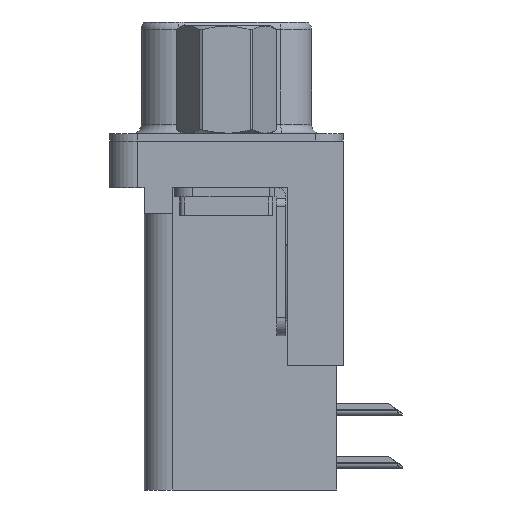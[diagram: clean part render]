
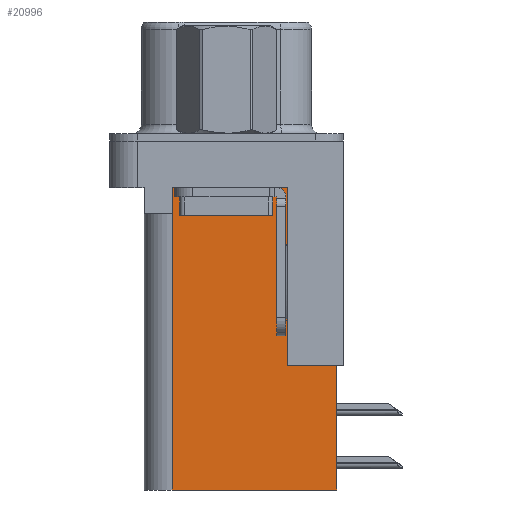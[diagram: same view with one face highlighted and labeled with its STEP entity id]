
A CAD part, left-side view. The second image highlights one B-rep face of the part: STEP entity #20996.
In plain terms, the highlighted planar face has unit normal (-1, 0, 0).
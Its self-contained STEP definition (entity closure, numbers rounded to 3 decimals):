
#457 = EDGE_CURVE ( 'NONE', #27743, #21307, #26429, .T. ) ;
#660 = VERTEX_POINT ( 'NONE', #13632 ) ;
#711 = VERTEX_POINT ( 'NONE', #24376 ) ;
#1078 = CARTESIAN_POINT ( 'NONE',  ( 3.7, 2.925, -18.76 ) ) ;
#1459 = AXIS2_PLACEMENT_3D ( 'NONE', #18763, #21174, #7488 ) ;
#1855 = VECTOR ( 'NONE', #3613, 1000. ) ;
#2042 = LINE ( 'NONE', #19699, #1855 ) ;
#2372 = EDGE_CURVE ( 'NONE', #21307, #18124, #27006, .T. ) ;
#2862 = CARTESIAN_POINT ( 'NONE',  ( 3.7, -3.295, -2.5 ) ) ;
#2954 = DIRECTION ( 'NONE',  ( 0., 1., 0. ) ) ;
#3613 = DIRECTION ( 'NONE',  ( 0., 0., 1. ) ) ;
#3670 = CARTESIAN_POINT ( 'NONE',  ( 3.7, 2.895, -3.9 ) ) ;
#4594 = CARTESIAN_POINT ( 'NONE',  ( 3.7, 2.895, -2.5 ) ) ;
#4873 = LINE ( 'NONE', #19616, #5215 ) ;
#5215 = VECTOR ( 'NONE', #12898, 1000. ) ;
#6386 = DIRECTION ( 'NONE',  ( 0., 0., 1. ) ) ;
#7466 = VECTOR ( 'NONE', #21422, 1000. ) ;
#7488 = DIRECTION ( 'NONE',  ( 0., 1., 0. ) ) ;
#7599 = VECTOR ( 'NONE', #6386, 1000. ) ;
#7620 = LINE ( 'NONE', #12539, #7466 ) ;
#7969 = VECTOR ( 'NONE', #12021, 1000. ) ;
#8003 = LINE ( 'NONE', #24543, #7599 ) ;
#8039 = ORIENTED_EDGE ( 'NONE', *, *, #20003, .T. ) ;
#8108 = LINE ( 'NONE', #14321, #7969 ) ;
#8858 = ORIENTED_EDGE ( 'NONE', *, *, #2372, .T. ) ;
#12021 = DIRECTION ( 'NONE',  ( 0., 0., -1. ) ) ;
#12539 = CARTESIAN_POINT ( 'NONE',  ( 3.7, -3.295, -2.5 ) ) ;
#12898 = DIRECTION ( 'NONE',  ( 0., 1., 0. ) ) ;
#13337 = CARTESIAN_POINT ( 'NONE',  ( 3.7, 2.895, -3.9 ) ) ;
#13632 = CARTESIAN_POINT ( 'NONE',  ( 3.7, -5.925, -12.05 ) ) ;
#13918 = ORIENTED_EDGE ( 'NONE', *, *, #20403, .T. ) ;
#13957 = DIRECTION ( 'NONE',  ( 0., 0., -1. ) ) ;
#14321 = CARTESIAN_POINT ( 'NONE',  ( 3.7, -5.925, -2. ) ) ;
#14632 = VERTEX_POINT ( 'NONE', #1078 ) ;
#15466 = VECTOR ( 'NONE', #2954, 1000. ) ;
#15905 = LINE ( 'NONE', #21329, #15466 ) ;
#17082 = EDGE_CURVE ( 'NONE', #14632, #18124, #8003, .T. ) ;
#18124 = VERTEX_POINT ( 'NONE', #27904 ) ;
#18763 = CARTESIAN_POINT ( 'NONE',  ( 3.7, -3.295, -18.76 ) ) ;
#18866 = PLANE ( 'NONE',  #1459 ) ;
#19029 = EDGE_CURVE ( 'NONE', #20529, #14632, #15905, .T. ) ;
#19595 = EDGE_CURVE ( 'NONE', #660, #20529, #8108, .T. ) ;
#19616 = CARTESIAN_POINT ( 'NONE',  ( 3.7, -6.295, -12.05 ) ) ;
#19680 = ORIENTED_EDGE ( 'NONE', *, *, #28126, .T. ) ;
#19699 = CARTESIAN_POINT ( 'NONE',  ( 3.7, -3.295, -18.76 ) ) ;
#20003 = EDGE_CURVE ( 'NONE', #660, #711, #4873, .T. ) ;
#20403 = EDGE_CURVE ( 'NONE', #711, #27944, #2042, .T. ) ;
#20526 = CARTESIAN_POINT ( 'NONE',  ( 3.7, 0., -3.9 ) ) ;
#20529 = VERTEX_POINT ( 'NONE', #24450 ) ;
#20996 = ADVANCED_FACE ( 'NONE', ( #25083 ), #18866, .F. ) ;
#21174 = DIRECTION ( 'NONE',  ( 1., 0., 0. ) ) ;
#21307 = VERTEX_POINT ( 'NONE', #3670 ) ;
#21329 = CARTESIAN_POINT ( 'NONE',  ( 3.7, -3.295, -18.76 ) ) ;
#21422 = DIRECTION ( 'NONE',  ( 0., 1., 0. ) ) ;
#22725 = ORIENTED_EDGE ( 'NONE', *, *, #19595, .F. ) ;
#24376 = CARTESIAN_POINT ( 'NONE',  ( 3.7, -3.295, -12.05 ) ) ;
#24450 = CARTESIAN_POINT ( 'NONE',  ( 3.7, -5.925, -18.76 ) ) ;
#24543 = CARTESIAN_POINT ( 'NONE',  ( 3.7, 2.925, -18.76 ) ) ;
#25059 = ORIENTED_EDGE ( 'NONE', *, *, #17082, .F. ) ;
#25083 = FACE_OUTER_BOUND ( 'NONE', #25382, .T. ) ;
#25382 = EDGE_LOOP ( 'NONE', ( #19680, #27335, #8858, #25059, #27259, #22725, #8039, #13918 ) ) ;
#25889 = VECTOR ( 'NONE', #13957, 1000. ) ;
#26429 = LINE ( 'NONE', #13337, #25889 ) ;
#26836 = DIRECTION ( 'NONE',  ( 0., 1., 0. ) ) ;
#26899 = VECTOR ( 'NONE', #26836, 1000. ) ;
#27006 = LINE ( 'NONE', #20526, #26899 ) ;
#27259 = ORIENTED_EDGE ( 'NONE', *, *, #19029, .F. ) ;
#27335 = ORIENTED_EDGE ( 'NONE', *, *, #457, .T. ) ;
#27743 = VERTEX_POINT ( 'NONE', #4594 ) ;
#27904 = CARTESIAN_POINT ( 'NONE',  ( 3.7, 2.925, -3.9 ) ) ;
#27944 = VERTEX_POINT ( 'NONE', #2862 ) ;
#28126 = EDGE_CURVE ( 'NONE', #27944, #27743, #7620, .T. ) ;
